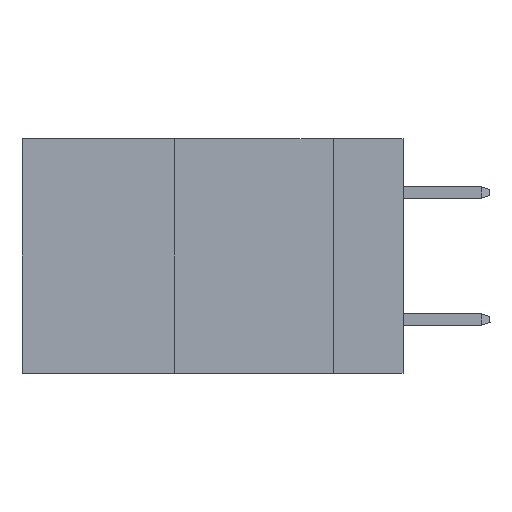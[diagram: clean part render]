
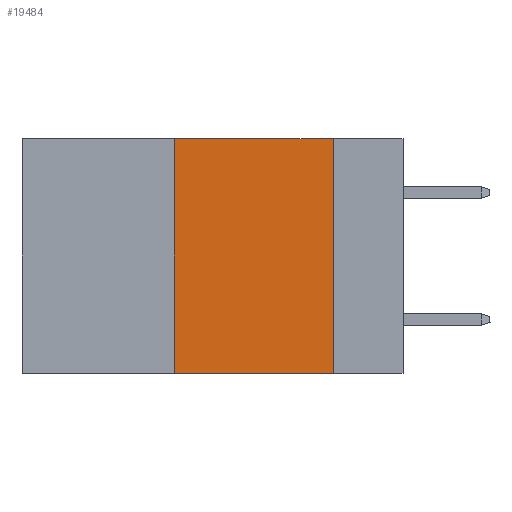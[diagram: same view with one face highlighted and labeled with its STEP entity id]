
A CAD part, left-side view. The second image highlights one B-rep face of the part: STEP entity #19484.
In plain terms, the highlighted planar face has unit normal (-1, 0, 0).
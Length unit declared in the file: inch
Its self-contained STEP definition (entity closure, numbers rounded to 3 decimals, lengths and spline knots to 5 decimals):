
#1782 = LINE ( 'NONE', #5132, #7806 ) ;
#1943 = CARTESIAN_POINT ( 'NONE',  ( 0., 0.6, 0. ) ) ;
#2706 = VERTEX_POINT ( 'NONE', #20066 ) ;
#3259 = LINE ( 'NONE', #19094, #16237 ) ;
#3519 = DIRECTION ( 'NONE',  ( 0., 0., -1. ) ) ;
#3885 = VERTEX_POINT ( 'NONE', #8952 ) ;
#4324 = EDGE_CURVE ( 'NONE', #14864, #16731, #3259, .T. ) ;
#5132 = CARTESIAN_POINT ( 'NONE',  ( 0., 0.11, 0. ) ) ;
#5472 = DIRECTION ( 'NONE',  ( 0., -1., 0. ) ) ;
#6091 = CARTESIAN_POINT ( 'NONE',  ( 0., 0.36, 0. ) ) ;
#6155 = EDGE_CURVE ( 'NONE', #14864, #2706, #6716, .T. ) ;
#6606 = EDGE_LOOP ( 'NONE', ( #16919, #7417, #14115, #16678 ) ) ;
#6657 = FACE_OUTER_BOUND ( 'NONE', #6606, .T. ) ;
#6716 = LINE ( 'NONE', #13128, #7377 ) ;
#7377 = VECTOR ( 'NONE', #13021, 39.37008 ) ;
#7417 = ORIENTED_EDGE ( 'NONE', *, *, #8772, .F. ) ;
#7806 = VECTOR ( 'NONE', #14079, 39.37008 ) ;
#8722 = LINE ( 'NONE', #13458, #12747 ) ;
#8772 = EDGE_CURVE ( 'NONE', #16731, #3885, #8722, .T. ) ;
#8952 = CARTESIAN_POINT ( 'NONE',  ( 0., 0.11, 0. ) ) ;
#11504 = PLANE ( 'NONE',  #13768 ) ;
#12060 = EDGE_CURVE ( 'NONE', #3885, #2706, #1782, .T. ) ;
#12747 = VECTOR ( 'NONE', #5472, 39.37008 ) ;
#13021 = DIRECTION ( 'NONE',  ( 0., -1., 0. ) ) ;
#13128 = CARTESIAN_POINT ( 'NONE',  ( 0., 0.6, -0.37 ) ) ;
#13458 = CARTESIAN_POINT ( 'NONE',  ( 0., 0.6, 0. ) ) ;
#13768 = AXIS2_PLACEMENT_3D ( 'NONE', #1943, #16311, #3519 ) ;
#14079 = DIRECTION ( 'NONE',  ( 0., 0., -1. ) ) ;
#14115 = ORIENTED_EDGE ( 'NONE', *, *, #4324, .F. ) ;
#14864 = VERTEX_POINT ( 'NONE', #15566 ) ;
#15566 = CARTESIAN_POINT ( 'NONE',  ( 0., 0.36, -0.37 ) ) ;
#16237 = VECTOR ( 'NONE', #20454, 39.37008 ) ;
#16311 = DIRECTION ( 'NONE',  ( 1., 0., 0. ) ) ;
#16678 = ORIENTED_EDGE ( 'NONE', *, *, #6155, .T. ) ;
#16731 = VERTEX_POINT ( 'NONE', #6091 ) ;
#16919 = ORIENTED_EDGE ( 'NONE', *, *, #12060, .F. ) ;
#19094 = CARTESIAN_POINT ( 'NONE',  ( 0., 0.36, 0. ) ) ;
#19484 = ADVANCED_FACE ( 'NONE', ( #6657 ), #11504, .F. ) ;
#20066 = CARTESIAN_POINT ( 'NONE',  ( 0., 0.11, -0.37 ) ) ;
#20454 = DIRECTION ( 'NONE',  ( 0., 0., 1. ) ) ;
